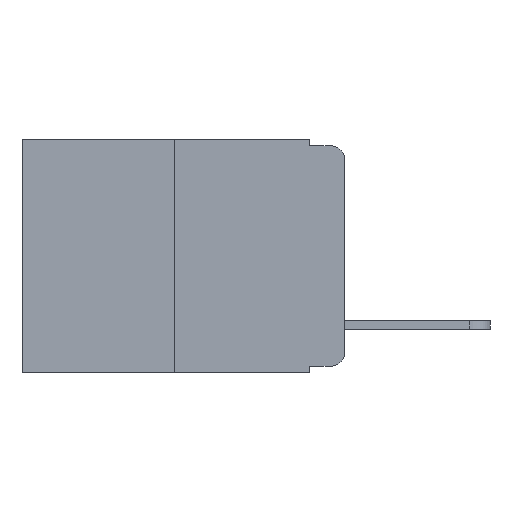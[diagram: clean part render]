
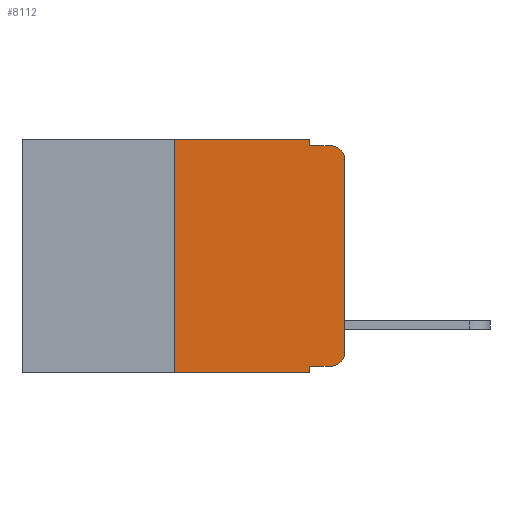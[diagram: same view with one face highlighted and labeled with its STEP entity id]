
A CAD part, left-side view. The second image highlights one B-rep face of the part: STEP entity #8112.
In plain terms, the highlighted planar face has unit normal (-1, 0, 0).
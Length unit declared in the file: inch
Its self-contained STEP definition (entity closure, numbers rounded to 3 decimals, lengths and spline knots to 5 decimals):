
#83 = LINE ( 'NONE', #299, #12334 ) ;
#113 = VERTEX_POINT ( 'NONE', #15661 ) ;
#299 = CARTESIAN_POINT ( 'NONE',  ( 0., 0.473, -0.343 ) ) ;
#354 = CARTESIAN_POINT ( 'NONE',  ( 0., 0., -0.03 ) ) ;
#425 = EDGE_CURVE ( 'NONE', #6660, #10502, #13159, .T. ) ;
#1266 = DIRECTION ( 'NONE',  ( 0., -1., 0. ) ) ;
#1359 = VECTOR ( 'NONE', #1266, 39.37008 ) ;
#1477 = VECTOR ( 'NONE', #6972, 39.37008 ) ;
#1889 = EDGE_CURVE ( 'NONE', #9805, #113, #83, .T. ) ;
#2017 = VECTOR ( 'NONE', #16281, 39.37008 ) ;
#2041 = VERTEX_POINT ( 'NONE', #16015 ) ;
#2792 = LINE ( 'NONE', #8859, #17986 ) ;
#3020 = EDGE_CURVE ( 'NONE', #10502, #18194, #10819, .T. ) ;
#3080 = ORIENTED_EDGE ( 'NONE', *, *, #17060, .T. ) ;
#3388 = VECTOR ( 'NONE', #3812, 39.37008 ) ;
#3632 = DIRECTION ( 'NONE',  ( 0., 0., -1. ) ) ;
#3801 = CARTESIAN_POINT ( 'NONE',  ( 0., 0.051, 0. ) ) ;
#3812 = DIRECTION ( 'NONE',  ( 0., 0., 1. ) ) ;
#4729 = ORIENTED_EDGE ( 'NONE', *, *, #425, .F. ) ;
#5012 = ORIENTED_EDGE ( 'NONE', *, *, #5972, .F. ) ;
#5381 = AXIS2_PLACEMENT_3D ( 'NONE', #14619, #13066, #9844 ) ;
#5498 = CARTESIAN_POINT ( 'NONE',  ( 0., 0., -0.313 ) ) ;
#5520 = CARTESIAN_POINT ( 'NONE',  ( 0., 0.051, -0.01 ) ) ;
#5844 = DIRECTION ( 'NONE',  ( 0., -1., 0. ) ) ;
#5972 = EDGE_CURVE ( 'NONE', #9805, #6660, #18142, .T. ) ;
#6205 = EDGE_CURVE ( 'NONE', #15950, #11746, #12538, .T. ) ;
#6419 = VERTEX_POINT ( 'NONE', #17349 ) ;
#6660 = VERTEX_POINT ( 'NONE', #10269 ) ;
#6866 = CARTESIAN_POINT ( 'NONE',  ( 0., 0., 0. ) ) ;
#6972 = DIRECTION ( 'NONE',  ( 0., 0., 1. ) ) ;
#7121 = ORIENTED_EDGE ( 'NONE', *, *, #15426, .F. ) ;
#7273 = CARTESIAN_POINT ( 'NONE',  ( 0., 0.02, -0.01 ) ) ;
#7613 = CARTESIAN_POINT ( 'NONE',  ( 0., 0.051, 0. ) ) ;
#7693 = ORIENTED_EDGE ( 'NONE', *, *, #16397, .T. ) ;
#8094 = DIRECTION ( 'NONE',  ( -1., 0., 0. ) ) ;
#8112 = ADVANCED_FACE ( 'NONE', ( #17809 ), #17468, .F. ) ;
#8196 = ORIENTED_EDGE ( 'NONE', *, *, #17499, .T. ) ;
#8440 = DIRECTION ( 'NONE',  ( 0., -1., 0. ) ) ;
#8501 = CARTESIAN_POINT ( 'NONE',  ( 0., 0.25, 0. ) ) ;
#8859 = CARTESIAN_POINT ( 'NONE',  ( 0., 0.051, -0.01 ) ) ;
#8882 = CIRCLE ( 'NONE', #5381, 0.02 ) ;
#9805 = VERTEX_POINT ( 'NONE', #15809 ) ;
#9844 = DIRECTION ( 'NONE',  ( 0., 0., -1. ) ) ;
#10269 = CARTESIAN_POINT ( 'NONE',  ( 0., 0.25, 0. ) ) ;
#10502 = VERTEX_POINT ( 'NONE', #7613 ) ;
#10819 = LINE ( 'NONE', #18539, #13259 ) ;
#10919 = EDGE_CURVE ( 'NONE', #6419, #113, #18894, .T. ) ;
#11019 = ORIENTED_EDGE ( 'NONE', *, *, #1889, .T. ) ;
#11283 = CARTESIAN_POINT ( 'NONE',  ( 0., 0.473, 0. ) ) ;
#11746 = VERTEX_POINT ( 'NONE', #354 ) ;
#11821 = CARTESIAN_POINT ( 'NONE',  ( 0., 0.473, 0. ) ) ;
#12053 = VERTEX_POINT ( 'NONE', #7273 ) ;
#12334 = VECTOR ( 'NONE', #18921, 39.37008 ) ;
#12538 = LINE ( 'NONE', #6866, #3388 ) ;
#12855 = DIRECTION ( 'NONE',  ( 1., 0., 0. ) ) ;
#13066 = DIRECTION ( 'NONE',  ( -1., 0., 0. ) ) ;
#13159 = LINE ( 'NONE', #11821, #1359 ) ;
#13217 = CARTESIAN_POINT ( 'NONE',  ( 0., 0.051, -0.333 ) ) ;
#13259 = VECTOR ( 'NONE', #13940, 39.37008 ) ;
#13791 = VECTOR ( 'NONE', #8440, 39.37008 ) ;
#13940 = DIRECTION ( 'NONE',  ( 0., 0., -1. ) ) ;
#14220 = CARTESIAN_POINT ( 'NONE',  ( 0., 0.02, -0.03 ) ) ;
#14425 = DIRECTION ( 'NONE',  ( 0., 0., -1. ) ) ;
#14523 = LINE ( 'NONE', #13217, #13791 ) ;
#14619 = CARTESIAN_POINT ( 'NONE',  ( 0., 0.02, -0.313 ) ) ;
#14631 = ORIENTED_EDGE ( 'NONE', *, *, #10919, .F. ) ;
#15130 = AXIS2_PLACEMENT_3D ( 'NONE', #11283, #12855, #3632 ) ;
#15426 = EDGE_CURVE ( 'NONE', #18194, #12053, #2792, .T. ) ;
#15661 = CARTESIAN_POINT ( 'NONE',  ( 0., 0.051, -0.343 ) ) ;
#15809 = CARTESIAN_POINT ( 'NONE',  ( 0., 0.25, -0.343 ) ) ;
#15950 = VERTEX_POINT ( 'NONE', #5498 ) ;
#16015 = CARTESIAN_POINT ( 'NONE',  ( 0., 0.02, -0.333 ) ) ;
#16266 = AXIS2_PLACEMENT_3D ( 'NONE', #14220, #8094, #14425 ) ;
#16281 = DIRECTION ( 'NONE',  ( 0., 0., -1. ) ) ;
#16397 = EDGE_CURVE ( 'NONE', #11746, #12053, #19594, .T. ) ;
#16752 = EDGE_LOOP ( 'NONE', ( #17741, #7693, #7121, #18146, #4729, #5012, #11019, #14631, #3080, #8196 ) ) ;
#17060 = EDGE_CURVE ( 'NONE', #6419, #2041, #14523, .T. ) ;
#17349 = CARTESIAN_POINT ( 'NONE',  ( 0., 0.051, -0.333 ) ) ;
#17468 = PLANE ( 'NONE',  #15130 ) ;
#17499 = EDGE_CURVE ( 'NONE', #2041, #15950, #8882, .T. ) ;
#17741 = ORIENTED_EDGE ( 'NONE', *, *, #6205, .T. ) ;
#17809 = FACE_OUTER_BOUND ( 'NONE', #16752, .T. ) ;
#17986 = VECTOR ( 'NONE', #5844, 39.37008 ) ;
#18142 = LINE ( 'NONE', #8501, #1477 ) ;
#18146 = ORIENTED_EDGE ( 'NONE', *, *, #3020, .F. ) ;
#18194 = VERTEX_POINT ( 'NONE', #5520 ) ;
#18539 = CARTESIAN_POINT ( 'NONE',  ( 0., 0.051, 0. ) ) ;
#18894 = LINE ( 'NONE', #3801, #2017 ) ;
#18921 = DIRECTION ( 'NONE',  ( 0., -1., 0. ) ) ;
#19594 = CIRCLE ( 'NONE', #16266, 0.02 ) ;
